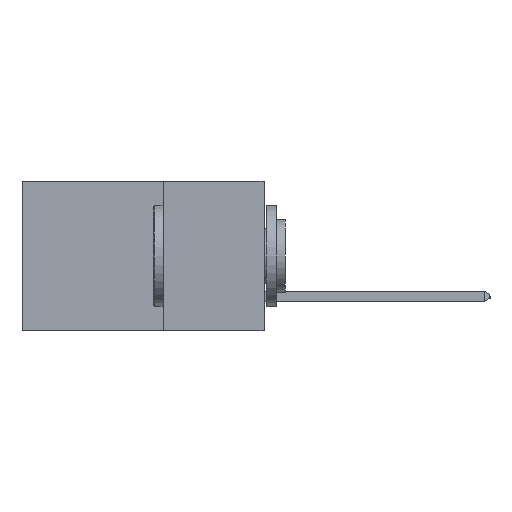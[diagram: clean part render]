
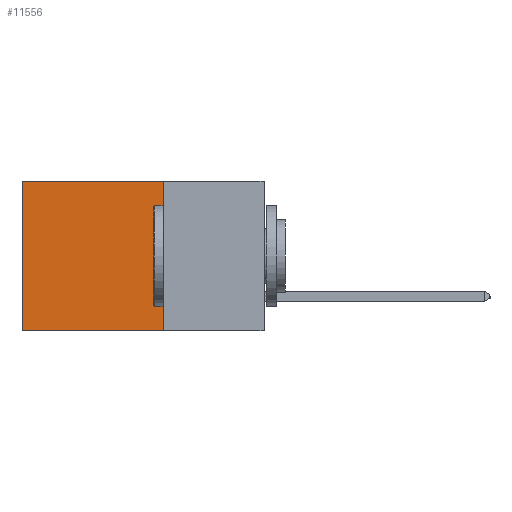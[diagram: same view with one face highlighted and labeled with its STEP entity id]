
A CAD part, left-side view. The second image highlights one B-rep face of the part: STEP entity #11556.
In plain terms, the highlighted planar face has unit normal (-1, 0, 0).
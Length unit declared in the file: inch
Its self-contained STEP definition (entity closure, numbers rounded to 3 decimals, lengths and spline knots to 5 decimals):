
#143 = AXIS2_PLACEMENT_3D ( 'NONE', #21299, #16048, #5274 ) ;
#395 = CARTESIAN_POINT ( 'NONE',  ( 0.298, 0.6, 0. ) ) ;
#1392 = DIRECTION ( 'NONE',  ( 0., 0., -1. ) ) ;
#1406 = LINE ( 'NONE', #21035, #15282 ) ;
#2097 = CARTESIAN_POINT ( 'NONE',  ( 0.298, 0.25, 0. ) ) ;
#2659 = EDGE_CURVE ( 'NONE', #11152, #9874, #1406, .T. ) ;
#3416 = PLANE ( 'NONE',  #143 ) ;
#3883 = LINE ( 'NONE', #2097, #21786 ) ;
#4005 = EDGE_CURVE ( 'NONE', #16370, #18680, #3883, .T. ) ;
#5274 = DIRECTION ( 'NONE',  ( 0., 0., -1. ) ) ;
#7019 = CARTESIAN_POINT ( 'NONE',  ( 0.298, 0.25, 0. ) ) ;
#7439 = EDGE_CURVE ( 'NONE', #18680, #9874, #7922, .T. ) ;
#7922 = LINE ( 'NONE', #14290, #16935 ) ;
#8990 = ORIENTED_EDGE ( 'NONE', *, *, #4005, .F. ) ;
#9066 = VECTOR ( 'NONE', #11966, 39.37008 ) ;
#9874 = VERTEX_POINT ( 'NONE', #14927 ) ;
#10143 = CARTESIAN_POINT ( 'NONE',  ( 0.298, 0.25, 0. ) ) ;
#11152 = VERTEX_POINT ( 'NONE', #395 ) ;
#11556 = ADVANCED_FACE ( 'NONE', ( #20696 ), #3416, .F. ) ;
#11966 = DIRECTION ( 'NONE',  ( 0., 1., 0. ) ) ;
#13128 = ORIENTED_EDGE ( 'NONE', *, *, #2659, .T. ) ;
#14061 = EDGE_LOOP ( 'NONE', ( #13128, #17896, #8990, #21457 ) ) ;
#14290 = CARTESIAN_POINT ( 'NONE',  ( 0.298, 0.25, -0.37 ) ) ;
#14370 = DIRECTION ( 'NONE',  ( 0., 1., 0. ) ) ;
#14927 = CARTESIAN_POINT ( 'NONE',  ( 0.298, 0.6, -0.37 ) ) ;
#15282 = VECTOR ( 'NONE', #1392, 39.37008 ) ;
#16048 = DIRECTION ( 'NONE',  ( 1., 0., 0. ) ) ;
#16370 = VERTEX_POINT ( 'NONE', #7019 ) ;
#16935 = VECTOR ( 'NONE', #14370, 39.37008 ) ;
#17896 = ORIENTED_EDGE ( 'NONE', *, *, #7439, .F. ) ;
#18488 = CARTESIAN_POINT ( 'NONE',  ( 0.298, 0.25, -0.37 ) ) ;
#18634 = LINE ( 'NONE', #10143, #9066 ) ;
#18680 = VERTEX_POINT ( 'NONE', #18488 ) ;
#20696 = FACE_OUTER_BOUND ( 'NONE', #14061, .T. ) ;
#21035 = CARTESIAN_POINT ( 'NONE',  ( 0.298, 0.6, 0. ) ) ;
#21299 = CARTESIAN_POINT ( 'NONE',  ( 0.298, 0.25, 0. ) ) ;
#21457 = ORIENTED_EDGE ( 'NONE', *, *, #22685, .T. ) ;
#21786 = VECTOR ( 'NONE', #22142, 39.37008 ) ;
#22142 = DIRECTION ( 'NONE',  ( 0., 0., -1. ) ) ;
#22685 = EDGE_CURVE ( 'NONE', #16370, #11152, #18634, .T. ) ;
